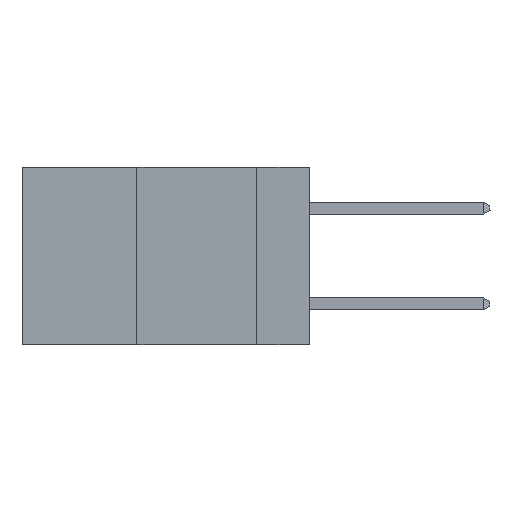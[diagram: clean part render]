
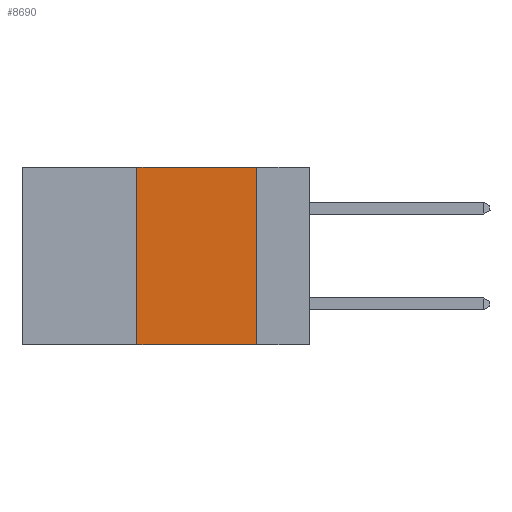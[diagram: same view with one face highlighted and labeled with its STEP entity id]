
A CAD part, left-side view. The second image highlights one B-rep face of the part: STEP entity #8690.
In plain terms, the highlighted planar face has unit normal (-1, 0, 0).
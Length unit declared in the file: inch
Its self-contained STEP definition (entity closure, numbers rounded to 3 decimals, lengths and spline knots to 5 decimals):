
#832 = VERTEX_POINT ( 'NONE', #6912 ) ;
#882 = DIRECTION ( 'NONE',  ( 0., 0., -1. ) ) ;
#1082 = CARTESIAN_POINT ( 'NONE',  ( 0., 0.36, 0. ) ) ;
#1230 = EDGE_CURVE ( 'NONE', #832, #4242, #5343, .T. ) ;
#1638 = ORIENTED_EDGE ( 'NONE', *, *, #1230, .F. ) ;
#1746 = PLANE ( 'NONE',  #6270 ) ;
#2291 = EDGE_CURVE ( 'NONE', #832, #8067, #3739, .T. ) ;
#2403 = EDGE_LOOP ( 'NONE', ( #5896, #9685, #1638, #9221 ) ) ;
#2636 = CARTESIAN_POINT ( 'NONE',  ( 0., 0.6, -0.37 ) ) ;
#2818 = VECTOR ( 'NONE', #8656, 39.37008 ) ;
#3052 = CARTESIAN_POINT ( 'NONE',  ( 0., 0.11, 0. ) ) ;
#3072 = DIRECTION ( 'NONE',  ( 0., -1., 0. ) ) ;
#3276 = VECTOR ( 'NONE', #5769, 39.37008 ) ;
#3280 = CARTESIAN_POINT ( 'NONE',  ( 0., 0.11, 0. ) ) ;
#3739 = LINE ( 'NONE', #2636, #3897 ) ;
#3897 = VECTOR ( 'NONE', #10270, 39.37008 ) ;
#4106 = FACE_OUTER_BOUND ( 'NONE', #2403, .T. ) ;
#4242 = VERTEX_POINT ( 'NONE', #1082 ) ;
#4389 = VERTEX_POINT ( 'NONE', #3052 ) ;
#4645 = LINE ( 'NONE', #10533, #8280 ) ;
#5328 = EDGE_CURVE ( 'NONE', #4242, #4389, #4645, .T. ) ;
#5343 = LINE ( 'NONE', #7635, #2818 ) ;
#5372 = CARTESIAN_POINT ( 'NONE',  ( 0., 0.11, -0.37 ) ) ;
#5769 = DIRECTION ( 'NONE',  ( 0., 0., -1. ) ) ;
#5896 = ORIENTED_EDGE ( 'NONE', *, *, #7284, .F. ) ;
#6270 = AXIS2_PLACEMENT_3D ( 'NONE', #9048, #8295, #882 ) ;
#6912 = CARTESIAN_POINT ( 'NONE',  ( 0., 0.36, -0.37 ) ) ;
#7284 = EDGE_CURVE ( 'NONE', #4389, #8067, #9655, .T. ) ;
#7635 = CARTESIAN_POINT ( 'NONE',  ( 0., 0.36, 0. ) ) ;
#8067 = VERTEX_POINT ( 'NONE', #5372 ) ;
#8280 = VECTOR ( 'NONE', #3072, 39.37008 ) ;
#8295 = DIRECTION ( 'NONE',  ( 1., 0., 0. ) ) ;
#8656 = DIRECTION ( 'NONE',  ( 0., 0., 1. ) ) ;
#8690 = ADVANCED_FACE ( 'NONE', ( #4106 ), #1746, .F. ) ;
#9048 = CARTESIAN_POINT ( 'NONE',  ( 0., 0.6, 0. ) ) ;
#9221 = ORIENTED_EDGE ( 'NONE', *, *, #2291, .T. ) ;
#9655 = LINE ( 'NONE', #3280, #3276 ) ;
#9685 = ORIENTED_EDGE ( 'NONE', *, *, #5328, .F. ) ;
#10270 = DIRECTION ( 'NONE',  ( 0., -1., 0. ) ) ;
#10533 = CARTESIAN_POINT ( 'NONE',  ( 0., 0.6, 0. ) ) ;
